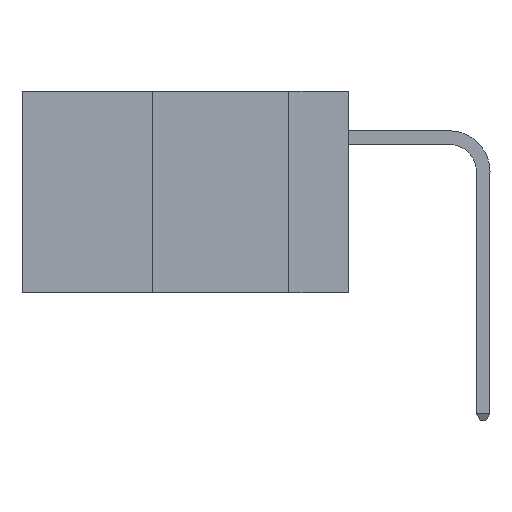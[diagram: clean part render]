
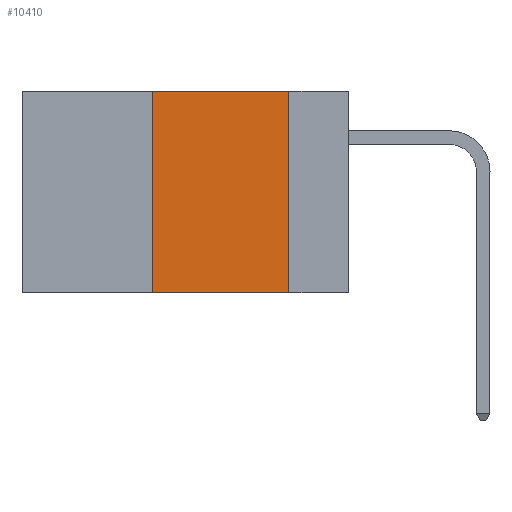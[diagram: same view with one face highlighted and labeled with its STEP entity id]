
A CAD part, left-side view. The second image highlights one B-rep face of the part: STEP entity #10410.
In plain terms, the highlighted planar face has unit normal (-1, 0, 0).
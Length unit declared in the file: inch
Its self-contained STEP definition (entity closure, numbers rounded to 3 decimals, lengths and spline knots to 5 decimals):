
#488 = CARTESIAN_POINT ( 'NONE',  ( 0., 0.6, 0. ) ) ;
#515 = DIRECTION ( 'NONE',  ( 0., 0., 1. ) ) ;
#1366 = LINE ( 'NONE', #10475, #9239 ) ;
#1554 = DIRECTION ( 'NONE',  ( 0., 0., -1. ) ) ;
#1732 = LINE ( 'NONE', #6305, #12313 ) ;
#1958 = VERTEX_POINT ( 'NONE', #7466 ) ;
#2065 = LINE ( 'NONE', #4795, #9906 ) ;
#2628 = CARTESIAN_POINT ( 'NONE',  ( 0., 0.36, 0. ) ) ;
#2666 = DIRECTION ( 'NONE',  ( 0., 0., -1. ) ) ;
#2750 = VERTEX_POINT ( 'NONE', #5853 ) ;
#4254 = ORIENTED_EDGE ( 'NONE', *, *, #5608, .F. ) ;
#4795 = CARTESIAN_POINT ( 'NONE',  ( 0., 0.11, 0. ) ) ;
#4967 = EDGE_CURVE ( 'NONE', #6558, #1958, #9753, .T. ) ;
#5172 = EDGE_CURVE ( 'NONE', #2750, #1958, #2065, .T. ) ;
#5224 = ORIENTED_EDGE ( 'NONE', *, *, #12120, .F. ) ;
#5428 = EDGE_LOOP ( 'NONE', ( #10450, #5224, #4254, #13080 ) ) ;
#5608 = EDGE_CURVE ( 'NONE', #6558, #12957, #1732, .T. ) ;
#5853 = CARTESIAN_POINT ( 'NONE',  ( 0., 0.11, 0. ) ) ;
#6305 = CARTESIAN_POINT ( 'NONE',  ( 0., 0.36, 0. ) ) ;
#6558 = VERTEX_POINT ( 'NONE', #6633 ) ;
#6633 = CARTESIAN_POINT ( 'NONE',  ( 0., 0.36, -0.37 ) ) ;
#7466 = CARTESIAN_POINT ( 'NONE',  ( 0., 0.11, -0.37 ) ) ;
#7722 = DIRECTION ( 'NONE',  ( 1., 0., 0. ) ) ;
#9239 = VECTOR ( 'NONE', #11516, 39.37008 ) ;
#9289 = FACE_OUTER_BOUND ( 'NONE', #5428, .T. ) ;
#9440 = VECTOR ( 'NONE', #9810, 39.37008 ) ;
#9753 = LINE ( 'NONE', #12142, #9440 ) ;
#9810 = DIRECTION ( 'NONE',  ( 0., -1., 0. ) ) ;
#9906 = VECTOR ( 'NONE', #2666, 39.37008 ) ;
#9940 = AXIS2_PLACEMENT_3D ( 'NONE', #488, #7722, #1554 ) ;
#10410 = ADVANCED_FACE ( 'NONE', ( #9289 ), #11784, .F. ) ;
#10450 = ORIENTED_EDGE ( 'NONE', *, *, #5172, .F. ) ;
#10475 = CARTESIAN_POINT ( 'NONE',  ( 0., 0.6, 0. ) ) ;
#11516 = DIRECTION ( 'NONE',  ( 0., -1., 0. ) ) ;
#11784 = PLANE ( 'NONE',  #9940 ) ;
#12120 = EDGE_CURVE ( 'NONE', #12957, #2750, #1366, .T. ) ;
#12142 = CARTESIAN_POINT ( 'NONE',  ( 0., 0.6, -0.37 ) ) ;
#12313 = VECTOR ( 'NONE', #515, 39.37008 ) ;
#12957 = VERTEX_POINT ( 'NONE', #2628 ) ;
#13080 = ORIENTED_EDGE ( 'NONE', *, *, #4967, .T. ) ;
